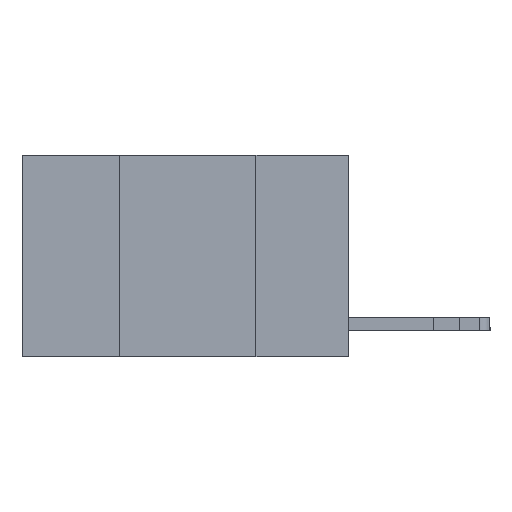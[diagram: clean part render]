
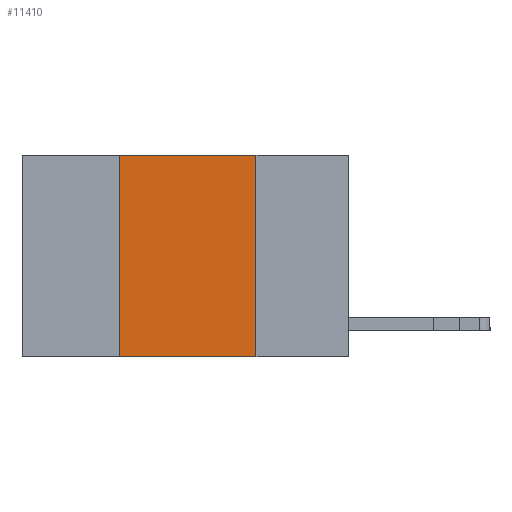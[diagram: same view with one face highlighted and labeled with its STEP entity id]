
A CAD part, left-side view. The second image highlights one B-rep face of the part: STEP entity #11410.
In plain terms, the highlighted planar face has unit normal (-1, 0, 0).
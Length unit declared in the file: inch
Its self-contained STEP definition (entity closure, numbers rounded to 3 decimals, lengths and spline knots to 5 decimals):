
#421 = DIRECTION ( 'NONE',  ( 1., 0., 0. ) ) ;
#1153 = EDGE_LOOP ( 'NONE', ( #5411, #12511, #9507, #2736 ) ) ;
#2282 = PLANE ( 'NONE',  #20749 ) ;
#2422 = VECTOR ( 'NONE', #3659, 39.37008 ) ;
#2736 = ORIENTED_EDGE ( 'NONE', *, *, #9104, .T. ) ;
#3225 = CARTESIAN_POINT ( 'NONE',  ( 0., 0.6, -0.37 ) ) ;
#3541 = VECTOR ( 'NONE', #15480, 39.37008 ) ;
#3552 = LINE ( 'NONE', #3225, #2422 ) ;
#3659 = DIRECTION ( 'NONE',  ( 0., -1., 0. ) ) ;
#3822 = VERTEX_POINT ( 'NONE', #10381 ) ;
#4351 = VERTEX_POINT ( 'NONE', #12332 ) ;
#4492 = EDGE_CURVE ( 'NONE', #21459, #3822, #9888, .T. ) ;
#4778 = LINE ( 'NONE', #16315, #19575 ) ;
#5411 = ORIENTED_EDGE ( 'NONE', *, *, #21220, .F. ) ;
#6274 = VECTOR ( 'NONE', #17931, 39.37008 ) ;
#7462 = CARTESIAN_POINT ( 'NONE',  ( 0., 0.6, 0. ) ) ;
#7747 = CARTESIAN_POINT ( 'NONE',  ( 0., 0.17, -0.37 ) ) ;
#8768 = LINE ( 'NONE', #20131, #3541 ) ;
#8984 = DIRECTION ( 'NONE',  ( 0., 0., -1. ) ) ;
#9104 = EDGE_CURVE ( 'NONE', #4351, #10166, #3552, .T. ) ;
#9507 = ORIENTED_EDGE ( 'NONE', *, *, #12508, .F. ) ;
#9888 = LINE ( 'NONE', #11200, #6274 ) ;
#10166 = VERTEX_POINT ( 'NONE', #7747 ) ;
#10263 = CARTESIAN_POINT ( 'NONE',  ( 0., 0.42, 0. ) ) ;
#10381 = CARTESIAN_POINT ( 'NONE',  ( 0., 0.17, 0. ) ) ;
#11200 = CARTESIAN_POINT ( 'NONE',  ( 0., 0.6, 0. ) ) ;
#11249 = DIRECTION ( 'NONE',  ( 0., 0., -1. ) ) ;
#11410 = ADVANCED_FACE ( 'NONE', ( #19035 ), #2282, .F. ) ;
#12332 = CARTESIAN_POINT ( 'NONE',  ( 0., 0.42, -0.37 ) ) ;
#12508 = EDGE_CURVE ( 'NONE', #4351, #21459, #8768, .T. ) ;
#12511 = ORIENTED_EDGE ( 'NONE', *, *, #4492, .F. ) ;
#15480 = DIRECTION ( 'NONE',  ( 0., 0., 1. ) ) ;
#16315 = CARTESIAN_POINT ( 'NONE',  ( 0., 0.17, 0. ) ) ;
#17931 = DIRECTION ( 'NONE',  ( 0., -1., 0. ) ) ;
#19035 = FACE_OUTER_BOUND ( 'NONE', #1153, .T. ) ;
#19575 = VECTOR ( 'NONE', #11249, 39.37008 ) ;
#20131 = CARTESIAN_POINT ( 'NONE',  ( 0., 0.42, 0. ) ) ;
#20749 = AXIS2_PLACEMENT_3D ( 'NONE', #7462, #421, #8984 ) ;
#21220 = EDGE_CURVE ( 'NONE', #3822, #10166, #4778, .T. ) ;
#21459 = VERTEX_POINT ( 'NONE', #10263 ) ;
